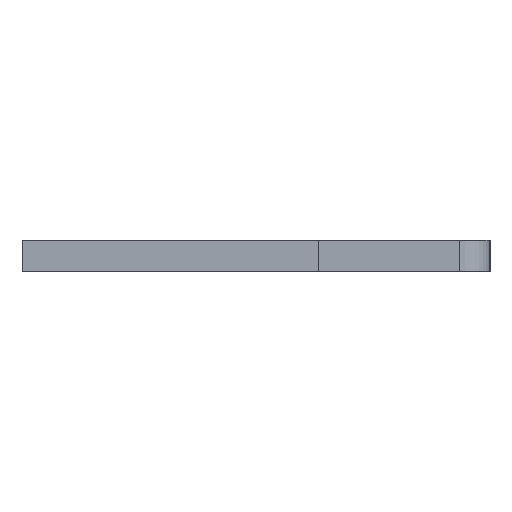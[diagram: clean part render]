
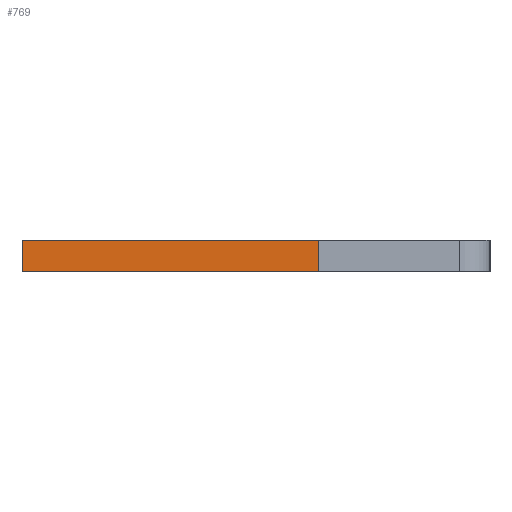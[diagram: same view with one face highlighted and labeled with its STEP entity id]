
A CAD part, left-side view. The second image highlights one B-rep face of the part: STEP entity #769.
In plain terms, the highlighted face is planar.
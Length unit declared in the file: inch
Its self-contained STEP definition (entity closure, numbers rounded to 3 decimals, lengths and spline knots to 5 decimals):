
#99 = VECTOR ( 'NONE', #226, 39.37008 ) ;
#113 = VECTOR ( 'NONE', #322, 39.37008 ) ;
#119 = CARTESIAN_POINT ( 'NONE',  ( 0.01, 0.15, -0.04 ) ) ;
#177 = CARTESIAN_POINT ( 'NONE',  ( 0.01, 0.15, -0.04 ) ) ;
#214 = CARTESIAN_POINT ( 'NONE',  ( 0.01, -0.04, -0.04 ) ) ;
#226 = DIRECTION ( 'NONE',  ( 0., 1., 0. ) ) ;
#235 = ORIENTED_EDGE ( 'NONE', *, *, #889, .T. ) ;
#251 = VERTEX_POINT ( 'NONE', #1012 ) ;
#286 = PLANE ( 'NONE',  #373 ) ;
#322 = DIRECTION ( 'NONE',  ( -1., 0., 0. ) ) ;
#351 = LINE ( 'NONE', #518, #99 ) ;
#373 = AXIS2_PLACEMENT_3D ( 'NONE', #177, #1018, #385 ) ;
#385 = DIRECTION ( 'NONE',  ( 1., 0., 0. ) ) ;
#412 = DIRECTION ( 'NONE',  ( 0., 1., 0. ) ) ;
#430 = ORIENTED_EDGE ( 'NONE', *, *, #931, .T. ) ;
#457 = EDGE_CURVE ( 'NONE', #251, #1086, #955, .T. ) ;
#518 = CARTESIAN_POINT ( 'NONE',  ( -0.01, 0.15, -0.04 ) ) ;
#530 = CARTESIAN_POINT ( 'NONE',  ( -0.01, -0.04, -0.04 ) ) ;
#566 = FACE_OUTER_BOUND ( 'NONE', #676, .T. ) ;
#676 = EDGE_LOOP ( 'NONE', ( #430, #923, #852, #235 ) ) ;
#769 = ADVANCED_FACE ( 'NONE', ( #566 ), #286, .F. ) ;
#852 = ORIENTED_EDGE ( 'NONE', *, *, #1109, .F. ) ;
#860 = LINE ( 'NONE', #1144, #113 ) ;
#889 = EDGE_CURVE ( 'NONE', #1137, #1156, #860, .T. ) ;
#923 = ORIENTED_EDGE ( 'NONE', *, *, #457, .F. ) ;
#931 = EDGE_CURVE ( 'NONE', #1156, #1086, #351, .T. ) ;
#955 = LINE ( 'NONE', #119, #1214 ) ;
#960 = CARTESIAN_POINT ( 'NONE',  ( 0.01, 0.15, -0.04 ) ) ;
#971 = LINE ( 'NONE', #960, #1050 ) ;
#1012 = CARTESIAN_POINT ( 'NONE',  ( 0.01, 0.15, -0.04 ) ) ;
#1018 = DIRECTION ( 'NONE',  ( 0., 0., 1. ) ) ;
#1036 = CARTESIAN_POINT ( 'NONE',  ( -0.01, 0.15, -0.04 ) ) ;
#1050 = VECTOR ( 'NONE', #412, 39.37008 ) ;
#1086 = VERTEX_POINT ( 'NONE', #1036 ) ;
#1109 = EDGE_CURVE ( 'NONE', #1137, #251, #971, .T. ) ;
#1137 = VERTEX_POINT ( 'NONE', #214 ) ;
#1144 = CARTESIAN_POINT ( 'NONE',  ( 0.01, -0.04, -0.04 ) ) ;
#1147 = DIRECTION ( 'NONE',  ( -1., 0., 0. ) ) ;
#1156 = VERTEX_POINT ( 'NONE', #530 ) ;
#1214 = VECTOR ( 'NONE', #1147, 39.37008 ) ;
